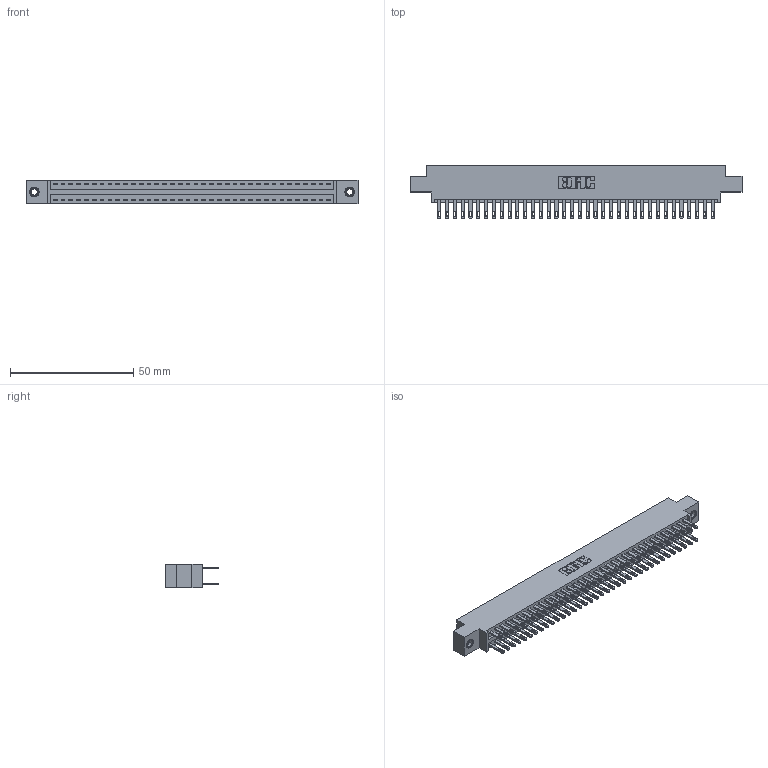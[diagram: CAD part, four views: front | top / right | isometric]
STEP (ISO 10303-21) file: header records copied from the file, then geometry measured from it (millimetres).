
FILE_DESCRIPTION (( 'STEP AP203' ), '1' );
FILE_NAME ('346-072-500-807.STEP', '2018-08-29T00:16:22', ( '' ), ( '' ), 'SwSTEP 2.0', 'SolidWorks 2016', '' );
FILE_SCHEMA (( 'CONFIG_CONTROL_DESIGN' ));
Length unit declared in the file: inch
Products named in the file (4): 346 Part_0.170 Offset - 0.156 Dia-TI; 345-292-001_345-293-100; 345-250-001_345-250-005-103; 346-072-500-807
Assembly tree (75 placements, depth 2):
  346-072-500-807
    346 Part_0.170 Offset - 0.156 Dia-TI
    345-292-001_345-293-100  x72
    345-250-001_345-250-005-103  x2
Bounding box: 134.87 x 21.84 x 9.4 mm (x, y, z)
Volume: 13157.2 mm3; surface area: 18958.1 mm2
Topology: 75 solids, 75 shells, 3642 faces, 11061 edges, 7366 vertices
Faces by surface type: plane 2200, cylinder 1426, cone 12, torus 4
Entity records: 25550 total; most frequent: CARTESIAN_POINT 4203, ORIENTED_EDGE 4130, DIRECTION 3783, EDGE_CURVE 2065, LINE 1765, VECTOR 1765, VERTEX_POINT 1372, AXIS2_PLACEMENT_3D 1009
